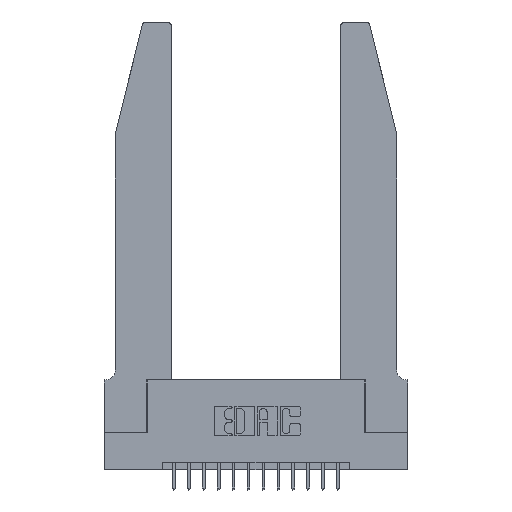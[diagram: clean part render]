
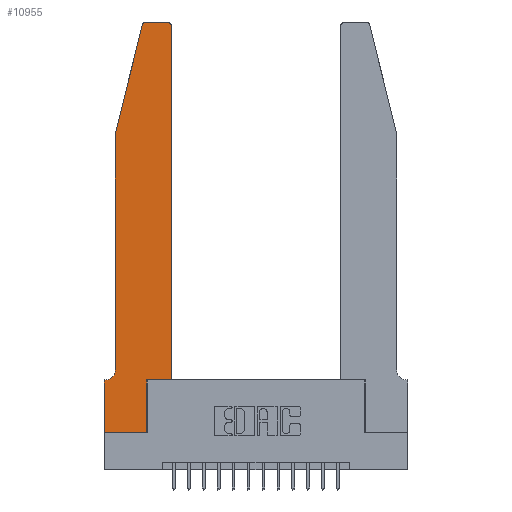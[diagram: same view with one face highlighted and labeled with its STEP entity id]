
A CAD part, top view. The second image highlights one B-rep face of the part: STEP entity #10955.
In plain terms, the highlighted planar face has unit normal (0, 0, 1).
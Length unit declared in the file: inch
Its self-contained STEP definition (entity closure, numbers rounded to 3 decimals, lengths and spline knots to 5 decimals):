
#18 = DIRECTION ( 'NONE',  ( -1., 0., 0. ) ) ;
#343 = ORIENTED_EDGE ( 'NONE', *, *, #6827, .T. ) ;
#598 = DIRECTION ( 'NONE',  ( -0.239, -0.971, 0. ) ) ;
#646 = VERTEX_POINT ( 'NONE', #4930 ) ;
#680 = ORIENTED_EDGE ( 'NONE', *, *, #17312, .T. ) ;
#752 = CARTESIAN_POINT ( 'NONE',  ( 0.2865, 0., 0.37 ) ) ;
#763 = EDGE_CURVE ( 'NONE', #14116, #15468, #14098, .T. ) ;
#851 = DIRECTION ( 'NONE',  ( 0., -1., 0. ) ) ;
#1048 = ORIENTED_EDGE ( 'NONE', *, *, #5819, .T. ) ;
#1170 = VECTOR ( 'NONE', #4467, 39.37008 ) ;
#1362 = AXIS2_PLACEMENT_3D ( 'NONE', #14217, #9850, #18 ) ;
#1484 = ORIENTED_EDGE ( 'NONE', *, *, #14445, .T. ) ;
#1567 = VERTEX_POINT ( 'NONE', #11780 ) ;
#1768 = CARTESIAN_POINT ( 'NONE',  ( 0.4505, 0.35, 0.37 ) ) ;
#1861 = ORIENTED_EDGE ( 'NONE', *, *, #7133, .T. ) ;
#2221 = VECTOR ( 'NONE', #9067, 39.37008 ) ;
#2301 = AXIS2_PLACEMENT_3D ( 'NONE', #12300, #5069, #9352 ) ;
#2956 = VERTEX_POINT ( 'NONE', #6603 ) ;
#3083 = CARTESIAN_POINT ( 'NONE',  ( 0., 0.35, 0.37 ) ) ;
#3207 = ORIENTED_EDGE ( 'NONE', *, *, #4773, .T. ) ;
#3380 = CARTESIAN_POINT ( 'NONE',  ( 0.2605, 2.75, 0.37 ) ) ;
#3532 = DIRECTION ( 'NONE',  ( 1., 0., 0. ) ) ;
#4467 = DIRECTION ( 'NONE',  ( 1., 0., 0. ) ) ;
#4762 = LINE ( 'NONE', #3380, #17598 ) ;
#4773 = EDGE_CURVE ( 'NONE', #15468, #16919, #6380, .T. ) ;
#4930 = CARTESIAN_POINT ( 'NONE',  ( 0.4505, 2.72, 0.37 ) ) ;
#4941 = DIRECTION ( 'NONE',  ( 1., 0., 0. ) ) ;
#4969 = LINE ( 'NONE', #16021, #18301 ) ;
#5069 = DIRECTION ( 'NONE',  ( 0., 0., 1. ) ) ;
#5326 = ORIENTED_EDGE ( 'NONE', *, *, #18009, .T. ) ;
#5819 = EDGE_CURVE ( 'NONE', #17699, #5954, #12847, .T. ) ;
#5954 = VERTEX_POINT ( 'NONE', #11294 ) ;
#6093 = ORIENTED_EDGE ( 'NONE', *, *, #763, .T. ) ;
#6183 = LINE ( 'NONE', #10444, #12586 ) ;
#6380 = LINE ( 'NONE', #13403, #10451 ) ;
#6603 = CARTESIAN_POINT ( 'NONE',  ( 0.0755, 0.42, 0.37 ) ) ;
#6650 = PLANE ( 'NONE',  #2301 ) ;
#6680 = AXIS2_PLACEMENT_3D ( 'NONE', #16074, #17535, #4941 ) ;
#6827 = EDGE_CURVE ( 'NONE', #7251, #14142, #6183, .T. ) ;
#7133 = EDGE_CURVE ( 'NONE', #1567, #17699, #4762, .T. ) ;
#7217 = VERTEX_POINT ( 'NONE', #9580 ) ;
#7251 = VERTEX_POINT ( 'NONE', #10026 ) ;
#7479 = CARTESIAN_POINT ( 'NONE',  ( 0.2865, 0.35, 0.37 ) ) ;
#7595 = ORIENTED_EDGE ( 'NONE', *, *, #13658, .T. ) ;
#7629 = DIRECTION ( 'NONE',  ( 0., 0., 1. ) ) ;
#7720 = LINE ( 'NONE', #1768, #11993 ) ;
#7787 = EDGE_CURVE ( 'NONE', #2956, #14116, #10842, .T. ) ;
#7838 = AXIS2_PLACEMENT_3D ( 'NONE', #13619, #7629, #3532 ) ;
#8549 = EDGE_CURVE ( 'NONE', #7217, #2956, #10704, .T. ) ;
#9067 = DIRECTION ( 'NONE',  ( 0., 1., 0. ) ) ;
#9251 = DIRECTION ( 'NONE',  ( 1., 0., 0. ) ) ;
#9314 = CARTESIAN_POINT ( 'NONE',  ( 0.0755, 2., 0.37 ) ) ;
#9352 = DIRECTION ( 'NONE',  ( 1., 0., 0. ) ) ;
#9532 = ORIENTED_EDGE ( 'NONE', *, *, #16539, .T. ) ;
#9579 = CARTESIAN_POINT ( 'NONE',  ( 0.4505, 0.35, 0.37 ) ) ;
#9580 = CARTESIAN_POINT ( 'NONE',  ( 0.0755, 2., 0.37 ) ) ;
#9763 = EDGE_LOOP ( 'NONE', ( #1861, #1048, #7595, #14664, #13262, #6093, #3207, #1484, #9532, #343, #680, #5326 ) ) ;
#9850 = DIRECTION ( 'NONE',  ( 0., 0., -1. ) ) ;
#10026 = CARTESIAN_POINT ( 'NONE',  ( 0.2865, 0.35, 0.37 ) ) ;
#10202 = LINE ( 'NONE', #17156, #1170 ) ;
#10248 = LINE ( 'NONE', #7479, #2221 ) ;
#10369 = DIRECTION ( 'NONE',  ( 0., -1., 0. ) ) ;
#10444 = CARTESIAN_POINT ( 'NONE',  ( 0.4505, 0.35, 0.37 ) ) ;
#10451 = VECTOR ( 'NONE', #10369, 39.37008 ) ;
#10704 = LINE ( 'NONE', #9314, #11731 ) ;
#10842 = CIRCLE ( 'NONE', #1362, 0.07 ) ;
#10955 = ADVANCED_FACE ( 'NONE', ( #12028 ), #6650, .T. ) ;
#11294 = CARTESIAN_POINT ( 'NONE',  ( 0.25487, 2.72718, 0.37 ) ) ;
#11731 = VECTOR ( 'NONE', #851, 39.37008 ) ;
#11776 = DIRECTION ( 'NONE',  ( 0., 1., 0. ) ) ;
#11780 = CARTESIAN_POINT ( 'NONE',  ( 0.4205, 2.75, 0.37 ) ) ;
#11993 = VECTOR ( 'NONE', #11776, 39.37008 ) ;
#12028 = FACE_OUTER_BOUND ( 'NONE', #9763, .T. ) ;
#12300 = CARTESIAN_POINT ( 'NONE',  ( 0., 0.35, 0.37 ) ) ;
#12586 = VECTOR ( 'NONE', #9251, 39.37008 ) ;
#12847 = CIRCLE ( 'NONE', #7838, 0.03 ) ;
#13158 = VERTEX_POINT ( 'NONE', #752 ) ;
#13262 = ORIENTED_EDGE ( 'NONE', *, *, #7787, .T. ) ;
#13354 = CARTESIAN_POINT ( 'NONE',  ( 0., 0., 0.37 ) ) ;
#13403 = CARTESIAN_POINT ( 'NONE',  ( 0., 0., 0.37 ) ) ;
#13619 = CARTESIAN_POINT ( 'NONE',  ( 0.284, 2.72, 0.37 ) ) ;
#13658 = EDGE_CURVE ( 'NONE', #5954, #7217, #4969, .T. ) ;
#14098 = LINE ( 'NONE', #14191, #14922 ) ;
#14116 = VERTEX_POINT ( 'NONE', #14683 ) ;
#14142 = VERTEX_POINT ( 'NONE', #9579 ) ;
#14191 = CARTESIAN_POINT ( 'NONE',  ( 0.0755, 0.35, 0.37 ) ) ;
#14217 = CARTESIAN_POINT ( 'NONE',  ( 0.0055, 0.42, 0.37 ) ) ;
#14445 = EDGE_CURVE ( 'NONE', #16919, #13158, #10202, .T. ) ;
#14664 = ORIENTED_EDGE ( 'NONE', *, *, #8549, .T. ) ;
#14683 = CARTESIAN_POINT ( 'NONE',  ( 0.0055, 0.35, 0.37 ) ) ;
#14686 = DIRECTION ( 'NONE',  ( -1., 0., 0. ) ) ;
#14922 = VECTOR ( 'NONE', #17060, 39.37008 ) ;
#14987 = CIRCLE ( 'NONE', #6680, 0.03 ) ;
#15261 = CARTESIAN_POINT ( 'NONE',  ( 0.284, 2.75, 0.37 ) ) ;
#15468 = VERTEX_POINT ( 'NONE', #3083 ) ;
#16021 = CARTESIAN_POINT ( 'NONE',  ( 0.0755, 2., 0.37 ) ) ;
#16074 = CARTESIAN_POINT ( 'NONE',  ( 0.4205, 2.72, 0.37 ) ) ;
#16539 = EDGE_CURVE ( 'NONE', #13158, #7251, #10248, .T. ) ;
#16919 = VERTEX_POINT ( 'NONE', #13354 ) ;
#17060 = DIRECTION ( 'NONE',  ( -1., 0., 0. ) ) ;
#17156 = CARTESIAN_POINT ( 'NONE',  ( 0., 0., 0.37 ) ) ;
#17312 = EDGE_CURVE ( 'NONE', #14142, #646, #7720, .T. ) ;
#17535 = DIRECTION ( 'NONE',  ( 0., 0., 1. ) ) ;
#17598 = VECTOR ( 'NONE', #14686, 39.37008 ) ;
#17699 = VERTEX_POINT ( 'NONE', #15261 ) ;
#18009 = EDGE_CURVE ( 'NONE', #646, #1567, #14987, .T. ) ;
#18301 = VECTOR ( 'NONE', #598, 39.37008 ) ;
